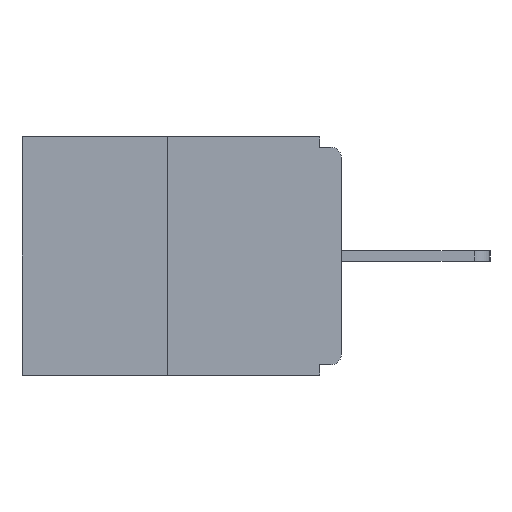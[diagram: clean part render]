
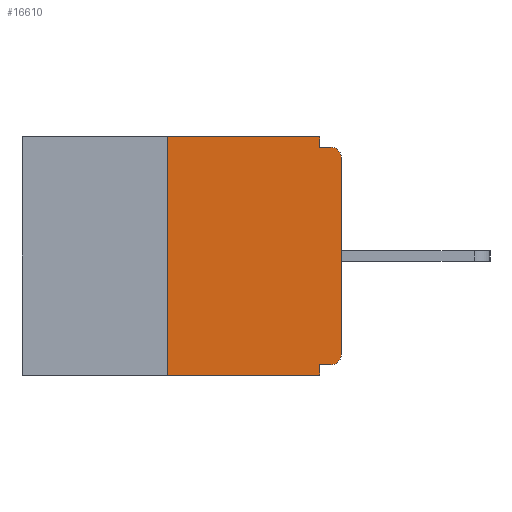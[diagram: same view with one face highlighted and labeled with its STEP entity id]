
A CAD part, left-side view. The second image highlights one B-rep face of the part: STEP entity #16610.
In plain terms, the highlighted planar face has unit normal (-1, 0, 0).
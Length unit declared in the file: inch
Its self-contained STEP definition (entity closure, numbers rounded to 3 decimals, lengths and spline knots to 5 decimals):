
#233 = DIRECTION ( 'NONE',  ( -1., 0., 0. ) ) ;
#257 = VERTEX_POINT ( 'NONE', #5774 ) ;
#321 = VECTOR ( 'NONE', #2485, 39.37008 ) ;
#559 = DIRECTION ( 'NONE',  ( 0., 0., -1. ) ) ;
#766 = CARTESIAN_POINT ( 'NONE',  ( 0., 0.031, 0. ) ) ;
#787 = DIRECTION ( 'NONE',  ( 0., -1., 0. ) ) ;
#1171 = CARTESIAN_POINT ( 'NONE',  ( 0., 0.015, -0.328 ) ) ;
#1443 = LINE ( 'NONE', #9376, #8275 ) ;
#1446 = EDGE_CURVE ( 'NONE', #1632, #11398, #15809, .T. ) ;
#1508 = DIRECTION ( 'NONE',  ( 0., 0., -1. ) ) ;
#1632 = VERTEX_POINT ( 'NONE', #6195 ) ;
#1678 = ORIENTED_EDGE ( 'NONE', *, *, #8266, .T. ) ;
#1715 = EDGE_CURVE ( 'NONE', #257, #11398, #14270, .T. ) ;
#2128 = AXIS2_PLACEMENT_3D ( 'NONE', #4126, #9292, #14502 ) ;
#2338 = CARTESIAN_POINT ( 'NONE',  ( 0., 0., -0.313 ) ) ;
#2371 = DIRECTION ( 'NONE',  ( 0., 0., -1. ) ) ;
#2485 = DIRECTION ( 'NONE',  ( 0., 0., -1. ) ) ;
#2541 = CARTESIAN_POINT ( 'NONE',  ( 0., 0.031, 0. ) ) ;
#3169 = VERTEX_POINT ( 'NONE', #7650 ) ;
#3223 = ORIENTED_EDGE ( 'NONE', *, *, #5976, .F. ) ;
#3337 = ORIENTED_EDGE ( 'NONE', *, *, #3776, .F. ) ;
#3341 = CIRCLE ( 'NONE', #11706, 0.015 ) ;
#3776 = EDGE_CURVE ( 'NONE', #11772, #7378, #4627, .T. ) ;
#4042 = DIRECTION ( 'NONE',  ( 0., -1., 0. ) ) ;
#4126 = CARTESIAN_POINT ( 'NONE',  ( 0., 0.46, 0. ) ) ;
#4627 = LINE ( 'NONE', #766, #7287 ) ;
#4680 = DIRECTION ( 'NONE',  ( 0., 0., 1. ) ) ;
#4701 = LINE ( 'NONE', #9872, #9919 ) ;
#4959 = CARTESIAN_POINT ( 'NONE',  ( 0., 0.25, 0. ) ) ;
#4994 = CARTESIAN_POINT ( 'NONE',  ( 0., 0.031, -0.343 ) ) ;
#5217 = AXIS2_PLACEMENT_3D ( 'NONE', #14219, #233, #1508 ) ;
#5220 = EDGE_CURVE ( 'NONE', #14653, #11772, #13751, .T. ) ;
#5774 = CARTESIAN_POINT ( 'NONE',  ( 0., 0.031, -0.328 ) ) ;
#5782 = CARTESIAN_POINT ( 'NONE',  ( 0., 0.015, -0.313 ) ) ;
#5906 = CARTESIAN_POINT ( 'NONE',  ( 0., 0.031, -0.015 ) ) ;
#5976 = EDGE_CURVE ( 'NONE', #1632, #14653, #7134, .T. ) ;
#6101 = ORIENTED_EDGE ( 'NONE', *, *, #5220, .F. ) ;
#6195 = CARTESIAN_POINT ( 'NONE',  ( 0., 0.25, -0.343 ) ) ;
#6495 = FACE_OUTER_BOUND ( 'NONE', #10191, .T. ) ;
#6965 = CARTESIAN_POINT ( 'NONE',  ( 0., 0., -0.03 ) ) ;
#7134 = LINE ( 'NONE', #16391, #16483 ) ;
#7287 = VECTOR ( 'NONE', #2371, 39.37008 ) ;
#7307 = LINE ( 'NONE', #10023, #12057 ) ;
#7378 = VERTEX_POINT ( 'NONE', #5906 ) ;
#7650 = CARTESIAN_POINT ( 'NONE',  ( 0., 0.015, -0.015 ) ) ;
#8048 = VECTOR ( 'NONE', #13526, 39.37008 ) ;
#8246 = ORIENTED_EDGE ( 'NONE', *, *, #16013, .T. ) ;
#8266 = EDGE_CURVE ( 'NONE', #15692, #15993, #3341, .T. ) ;
#8275 = VECTOR ( 'NONE', #4042, 39.37008 ) ;
#8309 = VERTEX_POINT ( 'NONE', #6965 ) ;
#8322 = ORIENTED_EDGE ( 'NONE', *, *, #1715, .F. ) ;
#8499 = ORIENTED_EDGE ( 'NONE', *, *, #10705, .T. ) ;
#9292 = DIRECTION ( 'NONE',  ( 1., 0., 0. ) ) ;
#9376 = CARTESIAN_POINT ( 'NONE',  ( 0., 0., -0.015 ) ) ;
#9592 = CARTESIAN_POINT ( 'NONE',  ( 0., 0.46, -0.343 ) ) ;
#9832 = ORIENTED_EDGE ( 'NONE', *, *, #15706, .F. ) ;
#9872 = CARTESIAN_POINT ( 'NONE',  ( 0., 0., -0.328 ) ) ;
#9919 = VECTOR ( 'NONE', #14994, 39.37008 ) ;
#10023 = CARTESIAN_POINT ( 'NONE',  ( 0., 0., 0. ) ) ;
#10172 = ORIENTED_EDGE ( 'NONE', *, *, #15404, .F. ) ;
#10191 = EDGE_LOOP ( 'NONE', ( #6101, #3223, #13522, #8322, #9832, #1678, #8246, #8499, #10172, #3337 ) ) ;
#10565 = PLANE ( 'NONE',  #2128 ) ;
#10705 = EDGE_CURVE ( 'NONE', #8309, #3169, #11681, .T. ) ;
#11398 = VERTEX_POINT ( 'NONE', #4994 ) ;
#11510 = CARTESIAN_POINT ( 'NONE',  ( 0., 0.031, -0.343 ) ) ;
#11681 = CIRCLE ( 'NONE', #5217, 0.015 ) ;
#11706 = AXIS2_PLACEMENT_3D ( 'NONE', #5782, #16066, #559 ) ;
#11772 = VERTEX_POINT ( 'NONE', #2541 ) ;
#12057 = VECTOR ( 'NONE', #4680, 39.37008 ) ;
#12271 = DIRECTION ( 'NONE',  ( 0., 0., 1. ) ) ;
#13522 = ORIENTED_EDGE ( 'NONE', *, *, #1446, .T. ) ;
#13526 = DIRECTION ( 'NONE',  ( 0., -1., 0. ) ) ;
#13751 = LINE ( 'NONE', #14779, #14301 ) ;
#14219 = CARTESIAN_POINT ( 'NONE',  ( 0., 0.015, -0.03 ) ) ;
#14270 = LINE ( 'NONE', #11510, #321 ) ;
#14301 = VECTOR ( 'NONE', #787, 39.37008 ) ;
#14502 = DIRECTION ( 'NONE',  ( 0., 0., -1. ) ) ;
#14653 = VERTEX_POINT ( 'NONE', #4959 ) ;
#14779 = CARTESIAN_POINT ( 'NONE',  ( 0., 0.46, 0. ) ) ;
#14994 = DIRECTION ( 'NONE',  ( 0., 1., 0. ) ) ;
#15404 = EDGE_CURVE ( 'NONE', #7378, #3169, #1443, .T. ) ;
#15692 = VERTEX_POINT ( 'NONE', #1171 ) ;
#15706 = EDGE_CURVE ( 'NONE', #15692, #257, #4701, .T. ) ;
#15809 = LINE ( 'NONE', #9592, #8048 ) ;
#15993 = VERTEX_POINT ( 'NONE', #2338 ) ;
#16013 = EDGE_CURVE ( 'NONE', #15993, #8309, #7307, .T. ) ;
#16066 = DIRECTION ( 'NONE',  ( -1., 0., 0. ) ) ;
#16391 = CARTESIAN_POINT ( 'NONE',  ( 0., 0.25, 0. ) ) ;
#16483 = VECTOR ( 'NONE', #12271, 39.37008 ) ;
#16610 = ADVANCED_FACE ( 'NONE', ( #6495 ), #10565, .F. ) ;
